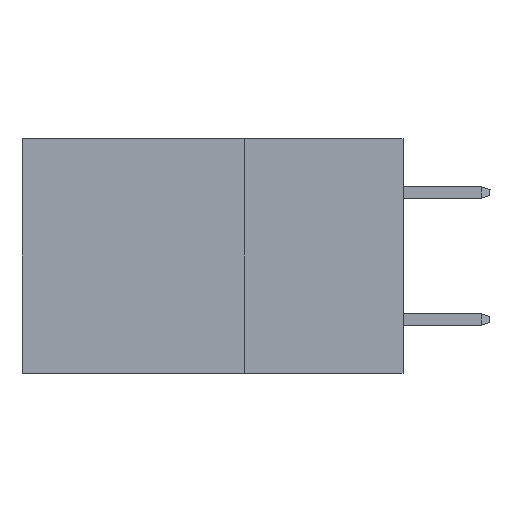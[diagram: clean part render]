
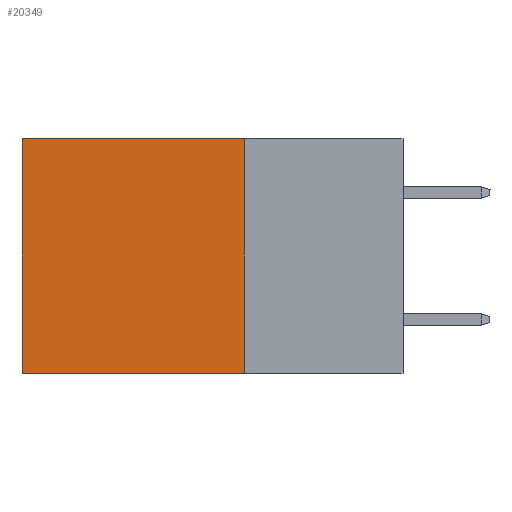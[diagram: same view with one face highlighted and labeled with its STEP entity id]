
A CAD part, left-side view. The second image highlights one B-rep face of the part: STEP entity #20349.
In plain terms, the highlighted planar face has unit normal (-1, 0, 0).
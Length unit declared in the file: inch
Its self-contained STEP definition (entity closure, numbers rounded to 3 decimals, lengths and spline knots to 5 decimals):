
#1048 = VECTOR ( 'NONE', #4095, 39.37008 ) ;
#1437 = VERTEX_POINT ( 'NONE', #9545 ) ;
#1748 = EDGE_CURVE ( 'NONE', #1437, #1833, #13379, .T. ) ;
#1833 = VERTEX_POINT ( 'NONE', #10866 ) ;
#2695 = CARTESIAN_POINT ( 'NONE',  ( 0.2875, 0.25, 0. ) ) ;
#2726 = EDGE_CURVE ( 'NONE', #4704, #1437, #6014, .T. ) ;
#3350 = CARTESIAN_POINT ( 'NONE',  ( 0.2875, 0.25, 0. ) ) ;
#3648 = DIRECTION ( 'NONE',  ( 0., 1., 0. ) ) ;
#4095 = DIRECTION ( 'NONE',  ( 0., 1., 0. ) ) ;
#4432 = ORIENTED_EDGE ( 'NONE', *, *, #18113, .T. ) ;
#4704 = VERTEX_POINT ( 'NONE', #6448 ) ;
#5171 = ORIENTED_EDGE ( 'NONE', *, *, #2726, .F. ) ;
#5923 = DIRECTION ( 'NONE',  ( 0., 0., -1. ) ) ;
#6014 = LINE ( 'NONE', #2695, #12067 ) ;
#6448 = CARTESIAN_POINT ( 'NONE',  ( 0.2875, 0.25, 0. ) ) ;
#9545 = CARTESIAN_POINT ( 'NONE',  ( 0.2875, 0.25, -0.37 ) ) ;
#9697 = ORIENTED_EDGE ( 'NONE', *, *, #16215, .T. ) ;
#10447 = PLANE ( 'NONE',  #14326 ) ;
#10644 = FACE_OUTER_BOUND ( 'NONE', #20260, .T. ) ;
#10866 = CARTESIAN_POINT ( 'NONE',  ( 0.2875, 0.6, -0.37 ) ) ;
#11154 = ORIENTED_EDGE ( 'NONE', *, *, #1748, .F. ) ;
#11903 = DIRECTION ( 'NONE',  ( 1., 0., 0. ) ) ;
#12005 = DIRECTION ( 'NONE',  ( 0., 0., -1. ) ) ;
#12067 = VECTOR ( 'NONE', #5923, 39.37008 ) ;
#13379 = LINE ( 'NONE', #16766, #1048 ) ;
#13486 = CARTESIAN_POINT ( 'NONE',  ( 0.2875, 0.25, 0. ) ) ;
#14326 = AXIS2_PLACEMENT_3D ( 'NONE', #13486, #11903, #12005 ) ;
#14818 = LINE ( 'NONE', #19753, #16336 ) ;
#15139 = VECTOR ( 'NONE', #3648, 39.37008 ) ;
#16215 = EDGE_CURVE ( 'NONE', #4704, #17751, #19382, .T. ) ;
#16336 = VECTOR ( 'NONE', #18477, 39.37008 ) ;
#16751 = CARTESIAN_POINT ( 'NONE',  ( 0.2875, 0.6, 0. ) ) ;
#16766 = CARTESIAN_POINT ( 'NONE',  ( 0.2875, 0.25, -0.37 ) ) ;
#17751 = VERTEX_POINT ( 'NONE', #16751 ) ;
#18113 = EDGE_CURVE ( 'NONE', #17751, #1833, #14818, .T. ) ;
#18477 = DIRECTION ( 'NONE',  ( 0., 0., -1. ) ) ;
#19382 = LINE ( 'NONE', #3350, #15139 ) ;
#19753 = CARTESIAN_POINT ( 'NONE',  ( 0.2875, 0.6, 0. ) ) ;
#20260 = EDGE_LOOP ( 'NONE', ( #4432, #11154, #5171, #9697 ) ) ;
#20349 = ADVANCED_FACE ( 'NONE', ( #10644 ), #10447, .F. ) ;
